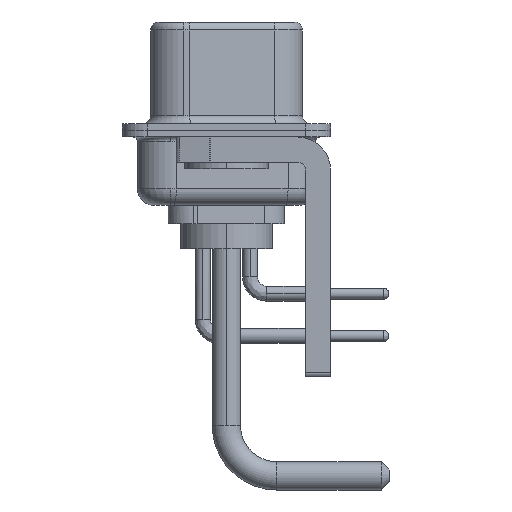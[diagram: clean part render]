
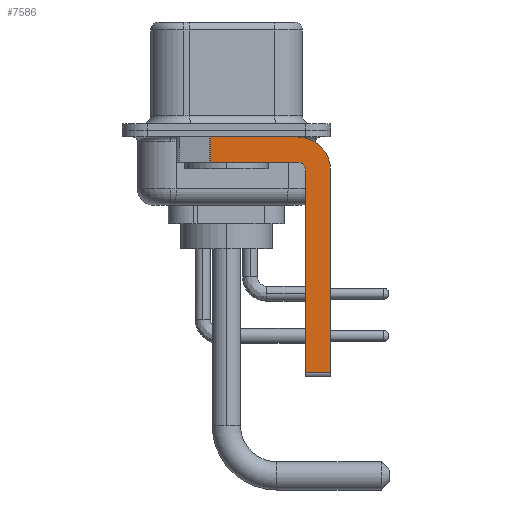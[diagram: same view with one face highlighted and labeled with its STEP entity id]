
A CAD part, left-side view. The second image highlights one B-rep face of the part: STEP entity #7586.
In plain terms, the highlighted planar face has unit normal (-1, 0, 0).
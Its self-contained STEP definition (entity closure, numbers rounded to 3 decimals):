
#320 = ORIENTED_EDGE ( 'NONE', *, *, #24248, .T. ) ;
#828 = VERTEX_POINT ( 'NONE', #3936 ) ;
#1912 = LINE ( 'NONE', #14304, #6491 ) ;
#2137 = EDGE_LOOP ( 'NONE', ( #18511, #320, #5628, #9910, #5398, #14854, #14053, #13597 ) ) ;
#2555 = CARTESIAN_POINT ( 'NONE',  ( -2.9, -4.25, -2.4 ) ) ;
#2995 = LINE ( 'NONE', #9461, #18091 ) ;
#3695 = VERTEX_POINT ( 'NONE', #16160 ) ;
#3936 = CARTESIAN_POINT ( 'NONE',  ( -2.9, -4.75, -14.55 ) ) ;
#5367 = CIRCLE ( 'NONE', #21824, 0.5 ) ;
#5398 = ORIENTED_EDGE ( 'NONE', *, *, #9530, .F. ) ;
#5628 = ORIENTED_EDGE ( 'NONE', *, *, #6730, .F. ) ;
#5724 = EDGE_CURVE ( 'NONE', #3695, #13891, #22209, .T. ) ;
#6352 = DIRECTION ( 'NONE',  ( 0., 0., -1. ) ) ;
#6412 = CARTESIAN_POINT ( 'NONE',  ( -2.9, -4.75, -14.8 ) ) ;
#6471 = DIRECTION ( 'NONE',  ( 1., 0., 0. ) ) ;
#6491 = VECTOR ( 'NONE', #21761, 1000. ) ;
#6670 = LINE ( 'NONE', #6412, #21754 ) ;
#6730 = EDGE_CURVE ( 'NONE', #13382, #17899, #1912, .T. ) ;
#6773 = CARTESIAN_POINT ( 'NONE',  ( -2.9, -4.25, -1.9 ) ) ;
#7586 = ADVANCED_FACE ( 'NONE', ( #16126 ), #9978, .F. ) ;
#7730 = AXIS2_PLACEMENT_3D ( 'NONE', #2555, #10451, #18294 ) ;
#8462 = CARTESIAN_POINT ( 'NONE',  ( -2.9, 0.978, -1.9 ) ) ;
#8531 = DIRECTION ( 'NONE',  ( 0., 0., 1. ) ) ;
#8948 = VECTOR ( 'NONE', #20288, 1000. ) ;
#9461 = CARTESIAN_POINT ( 'NONE',  ( -2.9, 3., -0.4 ) ) ;
#9530 = EDGE_CURVE ( 'NONE', #828, #14010, #6670, .T. ) ;
#9698 = LINE ( 'NONE', #23202, #20222 ) ;
#9910 = ORIENTED_EDGE ( 'NONE', *, *, #21486, .F. ) ;
#9978 = PLANE ( 'NONE',  #23412 ) ;
#10196 = EDGE_CURVE ( 'NONE', #12030, #10680, #2995, .T. ) ;
#10451 = DIRECTION ( 'NONE',  ( 1., 0., 0. ) ) ;
#10680 = VERTEX_POINT ( 'NONE', #19589 ) ;
#11629 = DIRECTION ( 'NONE',  ( 0., -1., 0. ) ) ;
#11905 = EDGE_CURVE ( 'NONE', #828, #13891, #9698, .T. ) ;
#12030 = VERTEX_POINT ( 'NONE', #18043 ) ;
#12563 = LINE ( 'NONE', #20399, #18192 ) ;
#13382 = VERTEX_POINT ( 'NONE', #6773 ) ;
#13597 = ORIENTED_EDGE ( 'NONE', *, *, #17024, .F. ) ;
#13891 = VERTEX_POINT ( 'NONE', #20381 ) ;
#14010 = VERTEX_POINT ( 'NONE', #23456 ) ;
#14053 = ORIENTED_EDGE ( 'NONE', *, *, #5724, .F. ) ;
#14304 = CARTESIAN_POINT ( 'NONE',  ( -2.9, -4.25, -1.9 ) ) ;
#14447 = CARTESIAN_POINT ( 'NONE',  ( -2.9, -4.25, -2.4 ) ) ;
#14689 = DIRECTION ( 'NONE',  ( -1., 0., 0. ) ) ;
#14737 = DIRECTION ( 'NONE',  ( 0., -1., 0. ) ) ;
#14854 = ORIENTED_EDGE ( 'NONE', *, *, #11905, .T. ) ;
#16126 = FACE_OUTER_BOUND ( 'NONE', #2137, .T. ) ;
#16160 = CARTESIAN_POINT ( 'NONE',  ( -2.9, -6.25, -2.4 ) ) ;
#17024 = EDGE_CURVE ( 'NONE', #10680, #3695, #24593, .T. ) ;
#17899 = VERTEX_POINT ( 'NONE', #8462 ) ;
#18043 = CARTESIAN_POINT ( 'NONE',  ( -2.9, 0.978, -0.4 ) ) ;
#18091 = VECTOR ( 'NONE', #14737, 1000. ) ;
#18192 = VECTOR ( 'NONE', #20002, 1000. ) ;
#18294 = DIRECTION ( 'NONE',  ( 0., 0., -1. ) ) ;
#18511 = ORIENTED_EDGE ( 'NONE', *, *, #10196, .F. ) ;
#19589 = CARTESIAN_POINT ( 'NONE',  ( -2.9, -4.25, -0.4 ) ) ;
#19897 = CARTESIAN_POINT ( 'NONE',  ( -2.9, -6.25, -2.4 ) ) ;
#20002 = DIRECTION ( 'NONE',  ( 0., 0., -1. ) ) ;
#20222 = VECTOR ( 'NONE', #11629, 1000. ) ;
#20288 = DIRECTION ( 'NONE',  ( 0., 0., -1. ) ) ;
#20381 = CARTESIAN_POINT ( 'NONE',  ( -2.9, -6.25, -14.55 ) ) ;
#20399 = CARTESIAN_POINT ( 'NONE',  ( -2.9, 0.978, -1.9 ) ) ;
#21486 = EDGE_CURVE ( 'NONE', #14010, #13382, #5367, .T. ) ;
#21754 = VECTOR ( 'NONE', #22623, 1000. ) ;
#21761 = DIRECTION ( 'NONE',  ( 0., 1., 0. ) ) ;
#21824 = AXIS2_PLACEMENT_3D ( 'NONE', #14447, #14689, #8531 ) ;
#22209 = LINE ( 'NONE', #19897, #8948 ) ;
#22623 = DIRECTION ( 'NONE',  ( 0., 0., 1. ) ) ;
#23202 = CARTESIAN_POINT ( 'NONE',  ( -2.9, -4.25, -14.55 ) ) ;
#23412 = AXIS2_PLACEMENT_3D ( 'NONE', #23997, #6471, #6352 ) ;
#23456 = CARTESIAN_POINT ( 'NONE',  ( -2.9, -4.75, -2.4 ) ) ;
#23997 = CARTESIAN_POINT ( 'NONE',  ( -2.9, -4.25, -2.4 ) ) ;
#24248 = EDGE_CURVE ( 'NONE', #12030, #17899, #12563, .T. ) ;
#24593 = CIRCLE ( 'NONE', #7730, 2. ) ;
